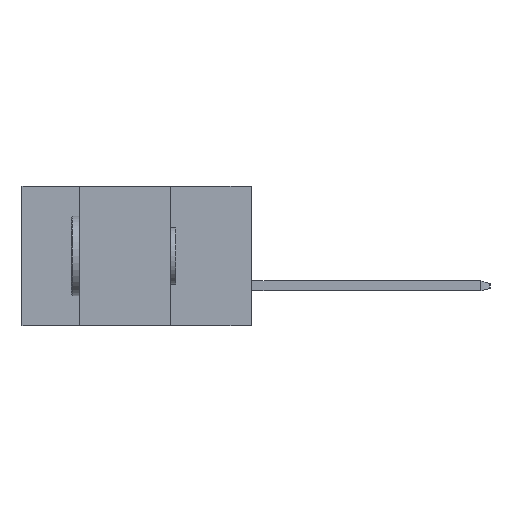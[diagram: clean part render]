
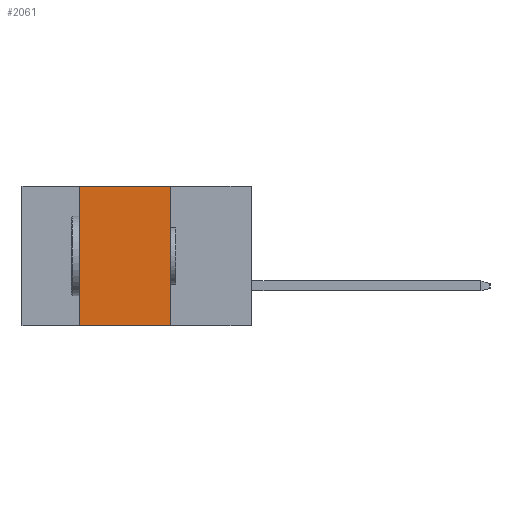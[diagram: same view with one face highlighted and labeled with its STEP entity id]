
A CAD part, left-side view. The second image highlights one B-rep face of the part: STEP entity #2061.
In plain terms, the highlighted planar face has unit normal (-1, 0, 0).
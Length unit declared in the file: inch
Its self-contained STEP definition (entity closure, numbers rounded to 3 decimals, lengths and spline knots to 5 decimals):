
#249 = EDGE_CURVE ( 'NONE', #6925, #10341, #7079, .T. ) ;
#556 = CARTESIAN_POINT ( 'NONE',  ( 0., 0.54, 0. ) ) ;
#773 = LINE ( 'NONE', #4451, #1619 ) ;
#859 = AXIS2_PLACEMENT_3D ( 'NONE', #7764, #5920, #7574 ) ;
#1039 = VERTEX_POINT ( 'NONE', #6153 ) ;
#1201 = EDGE_CURVE ( 'NONE', #6925, #1039, #773, .T. ) ;
#1619 = VECTOR ( 'NONE', #10128, 39.37008 ) ;
#1765 = EDGE_CURVE ( 'NONE', #4922, #1039, #11217, .T. ) ;
#1852 = DIRECTION ( 'NONE',  ( 0., 0., -1. ) ) ;
#2061 = ADVANCED_FACE ( 'NONE', ( #2200 ), #8555, .F. ) ;
#2200 = FACE_OUTER_BOUND ( 'NONE', #10433, .T. ) ;
#2709 = CARTESIAN_POINT ( 'NONE',  ( 0., 0.54, -0.437 ) ) ;
#3556 = VECTOR ( 'NONE', #10627, 39.37008 ) ;
#4127 = ORIENTED_EDGE ( 'NONE', *, *, #1201, .T. ) ;
#4451 = CARTESIAN_POINT ( 'NONE',  ( 0., 0.72, -0.437 ) ) ;
#4922 = VERTEX_POINT ( 'NONE', #5678 ) ;
#5057 = CARTESIAN_POINT ( 'NONE',  ( 0., 0.54, -0.437 ) ) ;
#5526 = EDGE_CURVE ( 'NONE', #10341, #4922, #9373, .T. ) ;
#5678 = CARTESIAN_POINT ( 'NONE',  ( 0., 0.254, 0. ) ) ;
#5920 = DIRECTION ( 'NONE',  ( 1., 0., 0. ) ) ;
#6153 = CARTESIAN_POINT ( 'NONE',  ( 0., 0.254, -0.437 ) ) ;
#6331 = ORIENTED_EDGE ( 'NONE', *, *, #5526, .F. ) ;
#6499 = DIRECTION ( 'NONE',  ( 0., -1., 0. ) ) ;
#6507 = CARTESIAN_POINT ( 'NONE',  ( 0., 0.254, -0.437 ) ) ;
#6925 = VERTEX_POINT ( 'NONE', #2709 ) ;
#7079 = LINE ( 'NONE', #5057, #3556 ) ;
#7574 = DIRECTION ( 'NONE',  ( 0., 0., -1. ) ) ;
#7764 = CARTESIAN_POINT ( 'NONE',  ( 0., 0.72, 0. ) ) ;
#8555 = PLANE ( 'NONE',  #859 ) ;
#9373 = LINE ( 'NONE', #10413, #12050 ) ;
#9853 = VECTOR ( 'NONE', #1852, 39.37008 ) ;
#10069 = ORIENTED_EDGE ( 'NONE', *, *, #249, .F. ) ;
#10128 = DIRECTION ( 'NONE',  ( 0., -1., 0. ) ) ;
#10341 = VERTEX_POINT ( 'NONE', #556 ) ;
#10413 = CARTESIAN_POINT ( 'NONE',  ( 0., 0.72, 0. ) ) ;
#10433 = EDGE_LOOP ( 'NONE', ( #11844, #6331, #10069, #4127 ) ) ;
#10627 = DIRECTION ( 'NONE',  ( 0., 0., 1. ) ) ;
#11217 = LINE ( 'NONE', #6507, #9853 ) ;
#11844 = ORIENTED_EDGE ( 'NONE', *, *, #1765, .F. ) ;
#12050 = VECTOR ( 'NONE', #6499, 39.37008 ) ;
